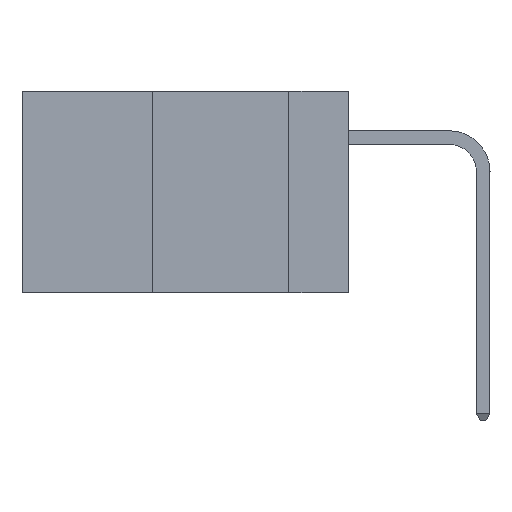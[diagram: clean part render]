
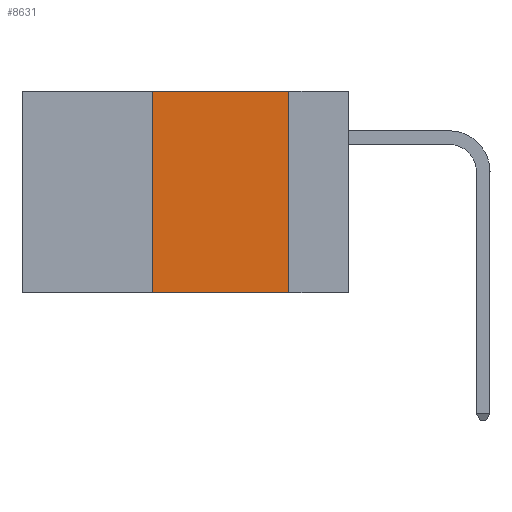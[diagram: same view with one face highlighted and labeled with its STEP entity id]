
A CAD part, left-side view. The second image highlights one B-rep face of the part: STEP entity #8631.
In plain terms, the highlighted planar face has unit normal (-1, 0, 0).
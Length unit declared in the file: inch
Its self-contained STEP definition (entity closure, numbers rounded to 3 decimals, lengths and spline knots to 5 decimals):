
#36 = LINE ( 'NONE', #22855, #22750 ) ;
#250 = CARTESIAN_POINT ( 'NONE',  ( 0., 0.36, 0. ) ) ;
#624 = CARTESIAN_POINT ( 'NONE',  ( 0., 0.36, -0.37 ) ) ;
#1786 = ORIENTED_EDGE ( 'NONE', *, *, #10517, .F. ) ;
#2412 = EDGE_LOOP ( 'NONE', ( #12036, #1786, #5095, #23097 ) ) ;
#2728 = DIRECTION ( 'NONE',  ( 1., 0., 0. ) ) ;
#2888 = CARTESIAN_POINT ( 'NONE',  ( 0., 0.11, 0. ) ) ;
#4190 = EDGE_CURVE ( 'NONE', #5393, #22599, #11375, .T. ) ;
#5095 = ORIENTED_EDGE ( 'NONE', *, *, #7580, .F. ) ;
#5178 = DIRECTION ( 'NONE',  ( 0., 0., -1. ) ) ;
#5393 = VERTEX_POINT ( 'NONE', #2888 ) ;
#5401 = FACE_OUTER_BOUND ( 'NONE', #2412, .T. ) ;
#7580 = EDGE_CURVE ( 'NONE', #21970, #8691, #16618, .T. ) ;
#8631 = ADVANCED_FACE ( 'NONE', ( #5401 ), #22770, .F. ) ;
#8691 = VERTEX_POINT ( 'NONE', #14202 ) ;
#10153 = LINE ( 'NONE', #17932, #23516 ) ;
#10517 = EDGE_CURVE ( 'NONE', #8691, #5393, #36, .T. ) ;
#10612 = CARTESIAN_POINT ( 'NONE',  ( 0., 0.11, 0. ) ) ;
#11375 = LINE ( 'NONE', #10612, #15653 ) ;
#11388 = DIRECTION ( 'NONE',  ( 0., 0., 1. ) ) ;
#12036 = ORIENTED_EDGE ( 'NONE', *, *, #4190, .F. ) ;
#13739 = CARTESIAN_POINT ( 'NONE',  ( 0., 0.6, 0. ) ) ;
#14202 = CARTESIAN_POINT ( 'NONE',  ( 0., 0.36, 0. ) ) ;
#15570 = DIRECTION ( 'NONE',  ( 0., 0., -1. ) ) ;
#15653 = VECTOR ( 'NONE', #5178, 39.37008 ) ;
#16044 = VECTOR ( 'NONE', #11388, 39.37008 ) ;
#16127 = DIRECTION ( 'NONE',  ( 0., -1., 0. ) ) ;
#16618 = LINE ( 'NONE', #250, #16044 ) ;
#17466 = DIRECTION ( 'NONE',  ( 0., -1., 0. ) ) ;
#17806 = EDGE_CURVE ( 'NONE', #21970, #22599, #10153, .T. ) ;
#17932 = CARTESIAN_POINT ( 'NONE',  ( 0., 0.6, -0.37 ) ) ;
#20245 = AXIS2_PLACEMENT_3D ( 'NONE', #13739, #2728, #15570 ) ;
#21970 = VERTEX_POINT ( 'NONE', #624 ) ;
#21973 = CARTESIAN_POINT ( 'NONE',  ( 0., 0.11, -0.37 ) ) ;
#22599 = VERTEX_POINT ( 'NONE', #21973 ) ;
#22750 = VECTOR ( 'NONE', #17466, 39.37008 ) ;
#22770 = PLANE ( 'NONE',  #20245 ) ;
#22855 = CARTESIAN_POINT ( 'NONE',  ( 0., 0.6, 0. ) ) ;
#23097 = ORIENTED_EDGE ( 'NONE', *, *, #17806, .T. ) ;
#23516 = VECTOR ( 'NONE', #16127, 39.37008 ) ;
